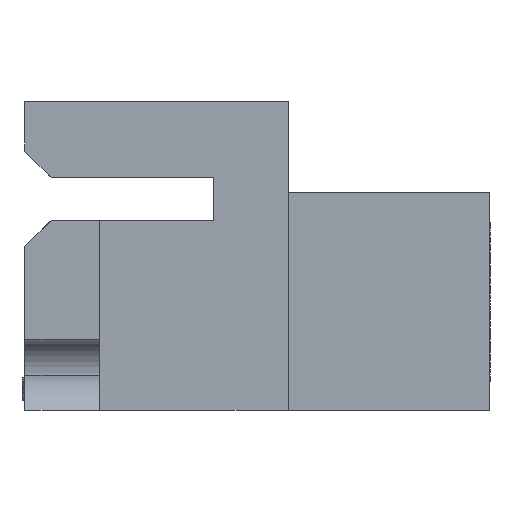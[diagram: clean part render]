
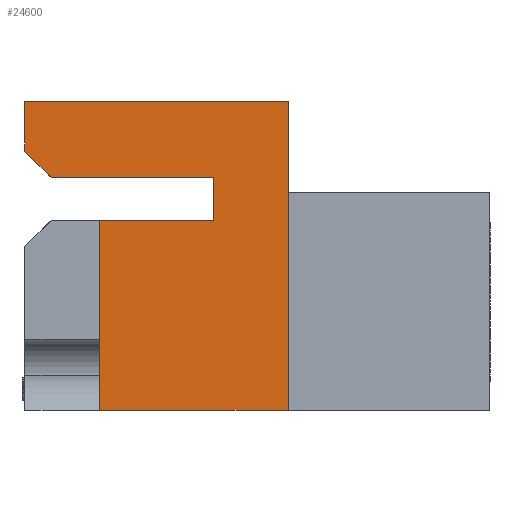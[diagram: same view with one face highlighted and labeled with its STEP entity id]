
A CAD part, left-side view. The second image highlights one B-rep face of the part: STEP entity #24600.
In plain terms, the highlighted planar face has unit normal (-1, 0, 0).
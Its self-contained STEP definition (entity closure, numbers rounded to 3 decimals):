
#88 = VECTOR ( 'NONE', #2913, 1000. ) ;
#137 = ORIENTED_EDGE ( 'NONE', *, *, #23282, .F. ) ;
#374 = ORIENTED_EDGE ( 'NONE', *, *, #31237, .F. ) ;
#1436 = DIRECTION ( 'NONE',  ( 0., 0., -1. ) ) ;
#1471 = EDGE_LOOP ( 'NONE', ( #26186, #31758, #35169, #28027, #9967, #19612, #137, #17539, #374 ) ) ;
#2201 = VERTEX_POINT ( 'NONE', #12194 ) ;
#2913 = DIRECTION ( 'NONE',  ( 0., 1., 0. ) ) ;
#6212 = VECTOR ( 'NONE', #30397, 1000. ) ;
#7219 = VERTEX_POINT ( 'NONE', #29330 ) ;
#7363 = DIRECTION ( 'NONE',  ( 0., 1., 0. ) ) ;
#7392 = LINE ( 'NONE', #27177, #14501 ) ;
#8832 = LINE ( 'NONE', #17280, #20398 ) ;
#9871 = LINE ( 'NONE', #31425, #88 ) ;
#9967 = ORIENTED_EDGE ( 'NONE', *, *, #36730, .T. ) ;
#10428 = EDGE_CURVE ( 'NONE', #34463, #2201, #26416, .T. ) ;
#11490 = VECTOR ( 'NONE', #7363, 1000. ) ;
#12194 = CARTESIAN_POINT ( 'NONE',  ( 0., 0., 0. ) ) ;
#12262 = VERTEX_POINT ( 'NONE', #19213 ) ;
#12311 = DIRECTION ( 'NONE',  ( 0., -1., 0. ) ) ;
#12411 = LINE ( 'NONE', #14572, #32050 ) ;
#12918 = VERTEX_POINT ( 'NONE', #18613 ) ;
#13160 = CARTESIAN_POINT ( 'NONE',  ( 0., 0., -5.182 ) ) ;
#13173 = CARTESIAN_POINT ( 'NONE',  ( 0., 11.506, -13.487 ) ) ;
#14501 = VECTOR ( 'NONE', #1436, 1000. ) ;
#14572 = CARTESIAN_POINT ( 'NONE',  ( 0., 8.255, -5.182 ) ) ;
#14879 = VERTEX_POINT ( 'NONE', #23980 ) ;
#15413 = FACE_OUTER_BOUND ( 'NONE', #1471, .T. ) ;
#15430 = CARTESIAN_POINT ( 'NONE',  ( 0., 0., 0. ) ) ;
#15602 = VERTEX_POINT ( 'NONE', #30783 ) ;
#17280 = CARTESIAN_POINT ( 'NONE',  ( 0., 3.251, -5.182 ) ) ;
#17539 = ORIENTED_EDGE ( 'NONE', *, *, #30109, .F. ) ;
#18613 = CARTESIAN_POINT ( 'NONE',  ( 0., 3.251, -3.302 ) ) ;
#18764 = EDGE_CURVE ( 'NONE', #2201, #34130, #7392, .T. ) ;
#19213 = CARTESIAN_POINT ( 'NONE',  ( 0., 3.251, -5.182 ) ) ;
#19612 = ORIENTED_EDGE ( 'NONE', *, *, #35850, .F. ) ;
#20125 = VERTEX_POINT ( 'NONE', #29767 ) ;
#20398 = VECTOR ( 'NONE', #22787, 1000. ) ;
#21162 = PLANE ( 'NONE',  #31707 ) ;
#22787 = DIRECTION ( 'NONE',  ( 0., 0., 1. ) ) ;
#22813 = DIRECTION ( 'NONE',  ( 0., 0., 1. ) ) ;
#23282 = EDGE_CURVE ( 'NONE', #12262, #12918, #8832, .T. ) ;
#23743 = CARTESIAN_POINT ( 'NONE',  ( 0., 0., -13.487 ) ) ;
#23980 = CARTESIAN_POINT ( 'NONE',  ( 0., 10.363, -3.302 ) ) ;
#24302 = DIRECTION ( 'NONE',  ( 0., 0., -1. ) ) ;
#24516 = DIRECTION ( 'NONE',  ( 0., -1., 0. ) ) ;
#24600 = ADVANCED_FACE ( 'NONE', ( #15413 ), #21162, .F. ) ;
#24867 = DIRECTION ( 'NONE',  ( 0., -0.707, -0.707 ) ) ;
#26186 = ORIENTED_EDGE ( 'NONE', *, *, #31396, .F. ) ;
#26416 = LINE ( 'NONE', #29127, #32649 ) ;
#26732 = VECTOR ( 'NONE', #24516, 1000. ) ;
#27162 = LINE ( 'NONE', #35685, #11490 ) ;
#27177 = CARTESIAN_POINT ( 'NONE',  ( 0., 0., 0. ) ) ;
#28027 = ORIENTED_EDGE ( 'NONE', *, *, #32330, .F. ) ;
#29127 = CARTESIAN_POINT ( 'NONE',  ( 0., 11.506, 0. ) ) ;
#29330 = CARTESIAN_POINT ( 'NONE',  ( 0., 8.255, -13.487 ) ) ;
#29767 = CARTESIAN_POINT ( 'NONE',  ( 0., 8.255, -5.182 ) ) ;
#30109 = EDGE_CURVE ( 'NONE', #20125, #12262, #34315, .T. ) ;
#30367 = CARTESIAN_POINT ( 'NONE',  ( 0., 10.363, -3.302 ) ) ;
#30397 = DIRECTION ( 'NONE',  ( 0., 0., 1. ) ) ;
#30783 = CARTESIAN_POINT ( 'NONE',  ( 0., 11.506, -2.159 ) ) ;
#30797 = LINE ( 'NONE', #13173, #6212 ) ;
#31058 = LINE ( 'NONE', #30367, #36002 ) ;
#31237 = EDGE_CURVE ( 'NONE', #7219, #20125, #12411, .T. ) ;
#31396 = EDGE_CURVE ( 'NONE', #34130, #7219, #27162, .T. ) ;
#31425 = CARTESIAN_POINT ( 'NONE',  ( 0., 0., -3.302 ) ) ;
#31707 = AXIS2_PLACEMENT_3D ( 'NONE', #15430, #35550, #24302 ) ;
#31758 = ORIENTED_EDGE ( 'NONE', *, *, #18764, .F. ) ;
#32050 = VECTOR ( 'NONE', #22813, 1000. ) ;
#32330 = EDGE_CURVE ( 'NONE', #15602, #34463, #30797, .T. ) ;
#32649 = VECTOR ( 'NONE', #12311, 1000. ) ;
#34130 = VERTEX_POINT ( 'NONE', #23743 ) ;
#34315 = LINE ( 'NONE', #13160, #26732 ) ;
#34463 = VERTEX_POINT ( 'NONE', #36040 ) ;
#35169 = ORIENTED_EDGE ( 'NONE', *, *, #10428, .F. ) ;
#35550 = DIRECTION ( 'NONE',  ( 1., 0., 0. ) ) ;
#35685 = CARTESIAN_POINT ( 'NONE',  ( 0., -8.814, -13.487 ) ) ;
#35850 = EDGE_CURVE ( 'NONE', #12918, #14879, #9871, .T. ) ;
#36002 = VECTOR ( 'NONE', #24867, 1000. ) ;
#36040 = CARTESIAN_POINT ( 'NONE',  ( 0., 11.506, 0. ) ) ;
#36730 = EDGE_CURVE ( 'NONE', #15602, #14879, #31058, .T. ) ;
